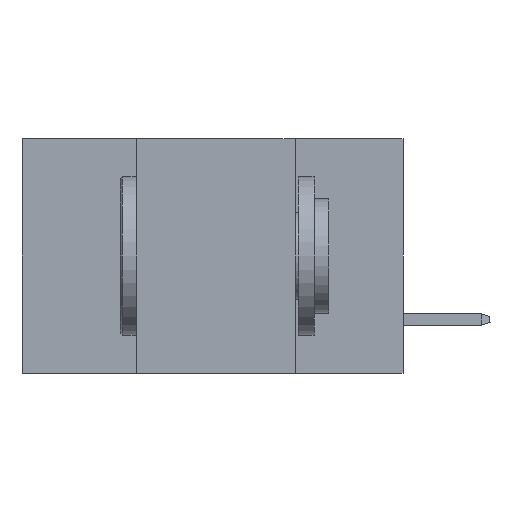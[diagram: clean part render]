
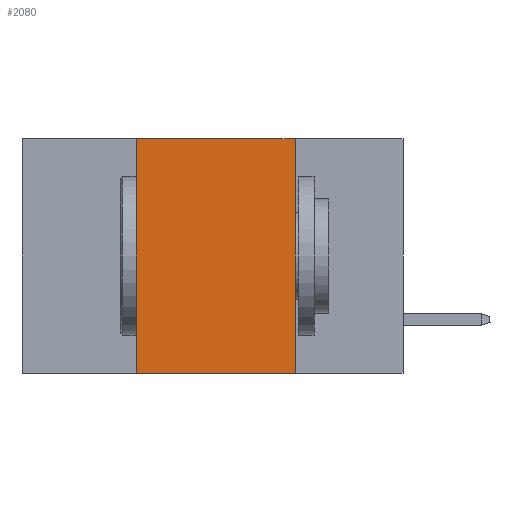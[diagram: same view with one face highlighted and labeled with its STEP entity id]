
A CAD part, left-side view. The second image highlights one B-rep face of the part: STEP entity #2080.
In plain terms, the highlighted planar face has unit normal (-1, 0, 0).
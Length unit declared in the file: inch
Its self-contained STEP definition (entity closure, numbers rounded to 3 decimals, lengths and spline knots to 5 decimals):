
#2029 = VECTOR ( 'NONE', #23121, 39.37008 ) ;
#2080 = ADVANCED_FACE ( 'NONE', ( #4657 ), #19605, .F. ) ;
#3054 = LINE ( 'NONE', #23275, #2029 ) ;
#3216 = DIRECTION ( 'NONE',  ( 0., 0., -1. ) ) ;
#3714 = ORIENTED_EDGE ( 'NONE', *, *, #28668, .T. ) ;
#4158 = EDGE_CURVE ( 'NONE', #32148, #14481, #15774, .T. ) ;
#4162 = DIRECTION ( 'NONE',  ( 0., 0., -1. ) ) ;
#4550 = VECTOR ( 'NONE', #26292, 39.37008 ) ;
#4657 = FACE_OUTER_BOUND ( 'NONE', #11489, .T. ) ;
#5923 = DIRECTION ( 'NONE',  ( 0., 0., 1. ) ) ;
#6110 = CARTESIAN_POINT ( 'NONE',  ( 0., 0.42, 0. ) ) ;
#6914 = ORIENTED_EDGE ( 'NONE', *, *, #23107, .F. ) ;
#8182 = VERTEX_POINT ( 'NONE', #14969 ) ;
#9723 = VECTOR ( 'NONE', #5923, 39.37008 ) ;
#10372 = CARTESIAN_POINT ( 'NONE',  ( 0., 0.42, 0. ) ) ;
#11489 = EDGE_LOOP ( 'NONE', ( #18434, #14786, #6914, #3714 ) ) ;
#11559 = CARTESIAN_POINT ( 'NONE',  ( 0., 0.6, 0. ) ) ;
#12431 = VERTEX_POINT ( 'NONE', #30969 ) ;
#14334 = DIRECTION ( 'NONE',  ( 1., 0., 0. ) ) ;
#14481 = VERTEX_POINT ( 'NONE', #22307 ) ;
#14582 = CARTESIAN_POINT ( 'NONE',  ( 0., 0.17, 0. ) ) ;
#14786 = ORIENTED_EDGE ( 'NONE', *, *, #4158, .F. ) ;
#14969 = CARTESIAN_POINT ( 'NONE',  ( 0., 0.42, -0.37 ) ) ;
#15774 = LINE ( 'NONE', #25816, #4550 ) ;
#16726 = AXIS2_PLACEMENT_3D ( 'NONE', #11559, #14334, #4162 ) ;
#18434 = ORIENTED_EDGE ( 'NONE', *, *, #31697, .F. ) ;
#19605 = PLANE ( 'NONE',  #16726 ) ;
#20471 = LINE ( 'NONE', #14582, #21906 ) ;
#21906 = VECTOR ( 'NONE', #3216, 39.37008 ) ;
#22307 = CARTESIAN_POINT ( 'NONE',  ( 0., 0.17, 0. ) ) ;
#23107 = EDGE_CURVE ( 'NONE', #8182, #32148, #25338, .T. ) ;
#23121 = DIRECTION ( 'NONE',  ( 0., -1., 0. ) ) ;
#23275 = CARTESIAN_POINT ( 'NONE',  ( 0., 0.6, -0.37 ) ) ;
#25338 = LINE ( 'NONE', #10372, #9723 ) ;
#25816 = CARTESIAN_POINT ( 'NONE',  ( 0., 0.6, 0. ) ) ;
#26292 = DIRECTION ( 'NONE',  ( 0., -1., 0. ) ) ;
#28668 = EDGE_CURVE ( 'NONE', #8182, #12431, #3054, .T. ) ;
#30969 = CARTESIAN_POINT ( 'NONE',  ( 0., 0.17, -0.37 ) ) ;
#31697 = EDGE_CURVE ( 'NONE', #14481, #12431, #20471, .T. ) ;
#32148 = VERTEX_POINT ( 'NONE', #6110 ) ;
